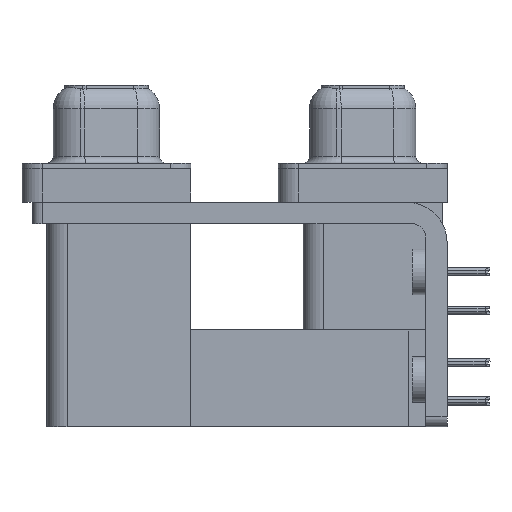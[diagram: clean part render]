
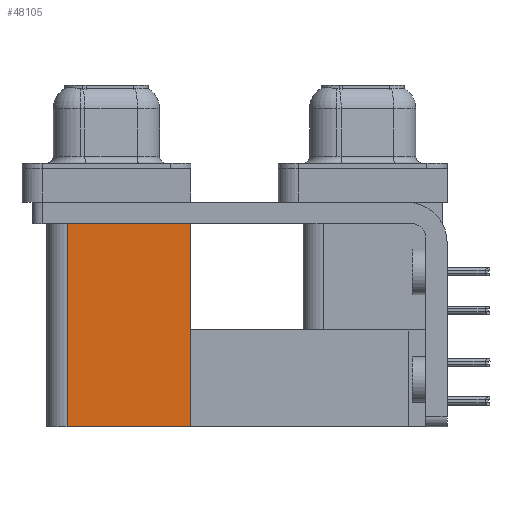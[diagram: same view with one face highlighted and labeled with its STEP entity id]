
A CAD part, left-side view. The second image highlights one B-rep face of the part: STEP entity #48105.
In plain terms, the highlighted planar face has unit normal (-1, 0, 0).
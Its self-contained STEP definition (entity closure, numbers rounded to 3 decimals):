
#1381 = VECTOR ( 'NONE', #27068, 1000. ) ;
#1792 = VECTOR ( 'NONE', #38036, 1000. ) ;
#3961 = VERTEX_POINT ( 'NONE', #28461 ) ;
#4251 = ORIENTED_EDGE ( 'NONE', *, *, #18672, .T. ) ;
#4309 = FACE_OUTER_BOUND ( 'NONE', #41023, .T. ) ;
#6882 = ORIENTED_EDGE ( 'NONE', *, *, #9446, .F. ) ;
#8194 = DIRECTION ( 'NONE',  ( 0., 0., 1. ) ) ;
#8440 = DIRECTION ( 'NONE',  ( 1., 0., 0. ) ) ;
#9161 = CARTESIAN_POINT ( 'NONE',  ( 3.765, 12.775, -19.2 ) ) ;
#9446 = EDGE_CURVE ( 'NONE', #34958, #18021, #46088, .T. ) ;
#11707 = ORIENTED_EDGE ( 'NONE', *, *, #32968, .T. ) ;
#11958 = CARTESIAN_POINT ( 'NONE',  ( 3.765, 21.975, -19.2 ) ) ;
#11970 = VECTOR ( 'NONE', #17321, 1000. ) ;
#12090 = CARTESIAN_POINT ( 'NONE',  ( 3.765, 12.775, -19.2 ) ) ;
#16230 = DIRECTION ( 'NONE',  ( 0., 0., -1. ) ) ;
#17321 = DIRECTION ( 'NONE',  ( 0., 1., 0. ) ) ;
#18021 = VERTEX_POINT ( 'NONE', #11958 ) ;
#18672 = EDGE_CURVE ( 'NONE', #34958, #3961, #27387, .T. ) ;
#19285 = LINE ( 'NONE', #46764, #1381 ) ;
#20112 = PLANE ( 'NONE',  #31679 ) ;
#20113 = EDGE_CURVE ( 'NONE', #18021, #42350, #19285, .T. ) ;
#27068 = DIRECTION ( 'NONE',  ( 0., 0., 1. ) ) ;
#27387 = LINE ( 'NONE', #12090, #29468 ) ;
#28395 = CARTESIAN_POINT ( 'NONE',  ( 3.765, 12.775, -19.2 ) ) ;
#28461 = CARTESIAN_POINT ( 'NONE',  ( 3.765, 12.775, -2.5 ) ) ;
#29468 = VECTOR ( 'NONE', #8194, 1000. ) ;
#31679 = AXIS2_PLACEMENT_3D ( 'NONE', #28395, #8440, #16230 ) ;
#32678 = CARTESIAN_POINT ( 'NONE',  ( 3.765, 21.975, -2.5 ) ) ;
#32968 = EDGE_CURVE ( 'NONE', #3961, #42350, #37501, .T. ) ;
#33114 = CARTESIAN_POINT ( 'NONE',  ( 3.765, 12.775, -2.5 ) ) ;
#34958 = VERTEX_POINT ( 'NONE', #9161 ) ;
#37501 = LINE ( 'NONE', #33114, #11970 ) ;
#38036 = DIRECTION ( 'NONE',  ( 0., 1., 0. ) ) ;
#40346 = ORIENTED_EDGE ( 'NONE', *, *, #20113, .F. ) ;
#41023 = EDGE_LOOP ( 'NONE', ( #11707, #40346, #6882, #4251 ) ) ;
#42350 = VERTEX_POINT ( 'NONE', #32678 ) ;
#46088 = LINE ( 'NONE', #50737, #1792 ) ;
#46764 = CARTESIAN_POINT ( 'NONE',  ( 3.765, 21.975, -19.2 ) ) ;
#48105 = ADVANCED_FACE ( 'NONE', ( #4309 ), #20112, .F. ) ;
#50737 = CARTESIAN_POINT ( 'NONE',  ( 3.765, 12.775, -19.2 ) ) ;
